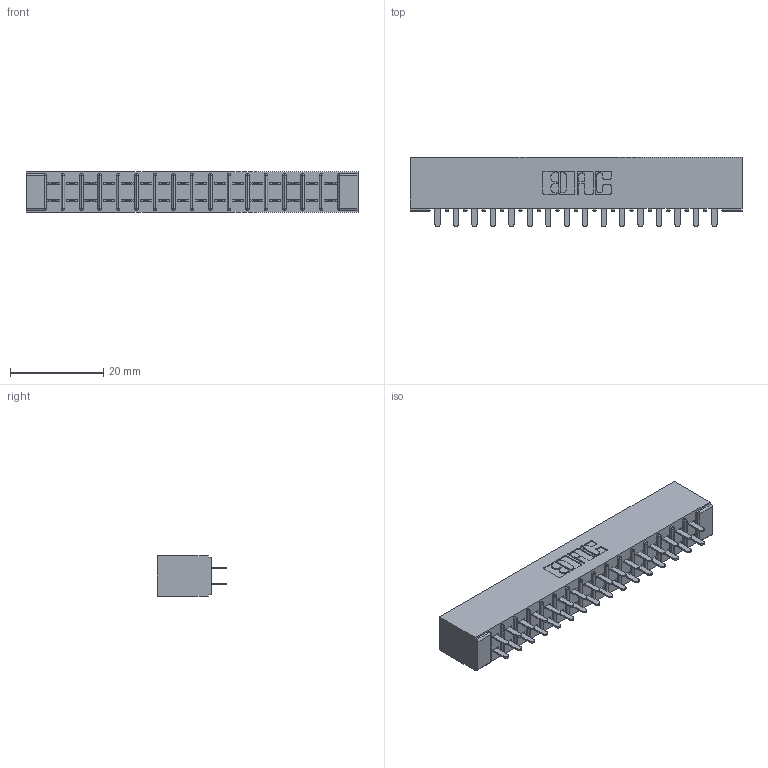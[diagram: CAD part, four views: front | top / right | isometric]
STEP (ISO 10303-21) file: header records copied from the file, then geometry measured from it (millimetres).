
FILE_DESCRIPTION (( 'STEP AP203' ), '1' );
FILE_NAME ('305-032-521-201.STEP', '2019-09-09T16:38:21', ( '' ), ( '' ), 'SwSTEP 2.0', 'SolidWorks 2016', '' );
FILE_SCHEMA (( 'CONFIG_CONTROL_DESIGN' ));
Length unit declared in the file: inch
Products named in the file (3): 305-032-521-201; 305 Part_No Mounting; 305-290-001_521
Assembly tree (33 placements, depth 2):
  305-032-521-201
    305 Part_No Mounting
    305-290-001_521  x32
Bounding box: 71.27 x 14.86 x 8.71 mm (x, y, z)
Volume: 4636.2 mm3; surface area: 8842.3 mm2
Topology: 33 solids, 33 shells, 1580 faces, 4500 edges, 2912 vertices
Faces by surface type: plane 928, cylinder 588, sphere 64
Entity records: 20091 total; most frequent: CARTESIAN_POINT 3322, ORIENTED_EDGE 3292, DIRECTION 3232, EDGE_CURVE 1646, LINE 1308, VECTOR 1308, VERTEX_POINT 1052, AXIS2_PLACEMENT_3D 962
